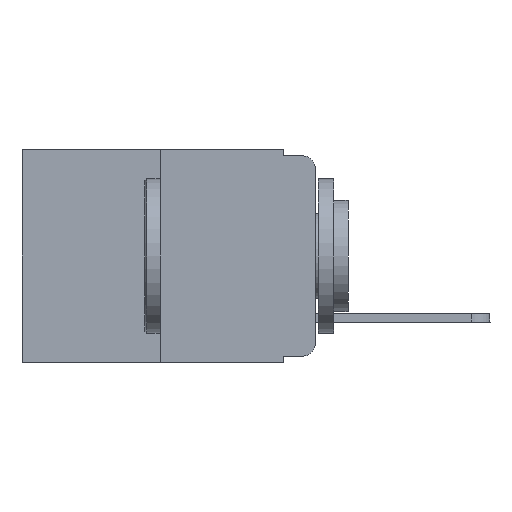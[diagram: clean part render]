
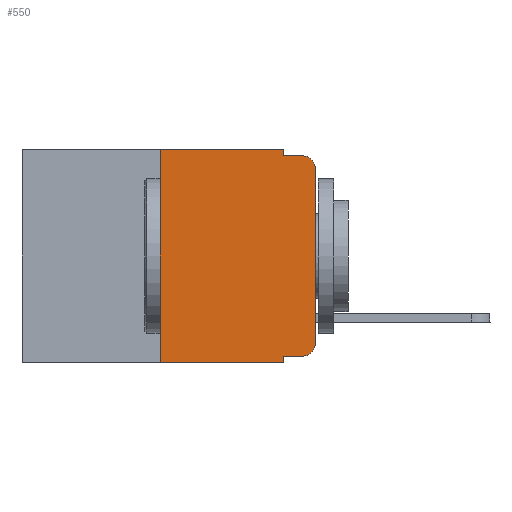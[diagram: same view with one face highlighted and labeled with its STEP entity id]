
A CAD part, left-side view. The second image highlights one B-rep face of the part: STEP entity #550.
In plain terms, the highlighted planar face has unit normal (-1, 0, 0).
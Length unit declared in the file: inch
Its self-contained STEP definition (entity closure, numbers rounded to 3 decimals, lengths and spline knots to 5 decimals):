
#314 = FACE_OUTER_BOUND ( 'NONE', #7585, .T. ) ;
#362 = DIRECTION ( 'NONE',  ( 0., 0., -1. ) ) ;
#365 = VERTEX_POINT ( 'NONE', #3191 ) ;
#460 = CIRCLE ( 'NONE', #5565, 0.02 ) ;
#550 = ADVANCED_FACE ( 'NONE', ( #314 ), #1403, .F. ) ;
#866 = DIRECTION ( 'NONE',  ( 0., 0., 1. ) ) ;
#910 = EDGE_CURVE ( 'NONE', #6566, #10781, #9144, .T. ) ;
#1000 = CARTESIAN_POINT ( 'NONE',  ( 0., 0.473, 0. ) ) ;
#1009 = EDGE_CURVE ( 'NONE', #2605, #8989, #460, .T. ) ;
#1221 = VERTEX_POINT ( 'NONE', #10163 ) ;
#1403 = PLANE ( 'NONE',  #7689 ) ;
#1728 = DIRECTION ( 'NONE',  ( 0., -1., 0. ) ) ;
#1851 = EDGE_CURVE ( 'NONE', #12961, #1221, #12371, .T. ) ;
#1961 = CARTESIAN_POINT ( 'NONE',  ( 0., 0.25, 0. ) ) ;
#2090 = DIRECTION ( 'NONE',  ( 0., -1., 0. ) ) ;
#2210 = VECTOR ( 'NONE', #2090, 39.37008 ) ;
#2278 = EDGE_CURVE ( 'NONE', #9634, #7809, #5179, .T. ) ;
#2605 = VERTEX_POINT ( 'NONE', #4623 ) ;
#2741 = CARTESIAN_POINT ( 'NONE',  ( 0., 0.473, -0.343 ) ) ;
#2773 = CARTESIAN_POINT ( 'NONE',  ( 0., 0.25, 0. ) ) ;
#2904 = CARTESIAN_POINT ( 'NONE',  ( 0., 0., -0.313 ) ) ;
#2907 = ORIENTED_EDGE ( 'NONE', *, *, #12034, .T. ) ;
#3114 = CARTESIAN_POINT ( 'NONE',  ( 0., 0.25, -0.343 ) ) ;
#3191 = CARTESIAN_POINT ( 'NONE',  ( 0., 0., -0.03 ) ) ;
#3356 = AXIS2_PLACEMENT_3D ( 'NONE', #10978, #5777, #4745 ) ;
#3427 = ORIENTED_EDGE ( 'NONE', *, *, #7143, .T. ) ;
#3485 = CARTESIAN_POINT ( 'NONE',  ( 0., 0.051, 0. ) ) ;
#3612 = DIRECTION ( 'NONE',  ( 0., 0., -1. ) ) ;
#3765 = ORIENTED_EDGE ( 'NONE', *, *, #4865, .F. ) ;
#3915 = LINE ( 'NONE', #3959, #11441 ) ;
#3959 = CARTESIAN_POINT ( 'NONE',  ( 0., 0.051, -0.333 ) ) ;
#4009 = CARTESIAN_POINT ( 'NONE',  ( 0., 0.051, 0. ) ) ;
#4623 = CARTESIAN_POINT ( 'NONE',  ( 0., 0.02, -0.333 ) ) ;
#4667 = DIRECTION ( 'NONE',  ( 1., 0., 0. ) ) ;
#4745 = DIRECTION ( 'NONE',  ( 0., 0., -1. ) ) ;
#4865 = EDGE_CURVE ( 'NONE', #7809, #6566, #5176, .T. ) ;
#5176 = LINE ( 'NONE', #1000, #2210 ) ;
#5179 = LINE ( 'NONE', #1961, #10401 ) ;
#5182 = ORIENTED_EDGE ( 'NONE', *, *, #1009, .T. ) ;
#5565 = AXIS2_PLACEMENT_3D ( 'NONE', #5571, #6618, #362 ) ;
#5571 = CARTESIAN_POINT ( 'NONE',  ( 0., 0.02, -0.313 ) ) ;
#5777 = DIRECTION ( 'NONE',  ( -1., 0., 0. ) ) ;
#5853 = VECTOR ( 'NONE', #6390, 39.37008 ) ;
#6011 = VECTOR ( 'NONE', #8711, 39.37008 ) ;
#6319 = VECTOR ( 'NONE', #11243, 39.37008 ) ;
#6356 = ORIENTED_EDGE ( 'NONE', *, *, #12206, .F. ) ;
#6390 = DIRECTION ( 'NONE',  ( 0., 0., 1. ) ) ;
#6396 = ORIENTED_EDGE ( 'NONE', *, *, #1851, .F. ) ;
#6566 = VERTEX_POINT ( 'NONE', #13171 ) ;
#6618 = DIRECTION ( 'NONE',  ( -1., 0., 0. ) ) ;
#6968 = ORIENTED_EDGE ( 'NONE', *, *, #10096, .T. ) ;
#7143 = EDGE_CURVE ( 'NONE', #365, #11783, #8053, .T. ) ;
#7462 = LINE ( 'NONE', #11970, #10920 ) ;
#7585 = EDGE_LOOP ( 'NONE', ( #2907, #3427, #6356, #13407, #3765, #7840, #6968, #6396, #12524, #5182 ) ) ;
#7689 = AXIS2_PLACEMENT_3D ( 'NONE', #11916, #4667, #3612 ) ;
#7809 = VERTEX_POINT ( 'NONE', #2773 ) ;
#7840 = ORIENTED_EDGE ( 'NONE', *, *, #2278, .F. ) ;
#8053 = CIRCLE ( 'NONE', #3356, 0.02 ) ;
#8711 = DIRECTION ( 'NONE',  ( 0., 0., -1. ) ) ;
#8807 = DIRECTION ( 'NONE',  ( 0., -1., 0. ) ) ;
#8965 = LINE ( 'NONE', #10591, #5853 ) ;
#8989 = VERTEX_POINT ( 'NONE', #2904 ) ;
#9144 = LINE ( 'NONE', #3485, #6011 ) ;
#9486 = EDGE_CURVE ( 'NONE', #12961, #2605, #3915, .T. ) ;
#9634 = VERTEX_POINT ( 'NONE', #3114 ) ;
#10067 = CARTESIAN_POINT ( 'NONE',  ( 0., 0.02, -0.01 ) ) ;
#10096 = EDGE_CURVE ( 'NONE', #9634, #1221, #10414, .T. ) ;
#10163 = CARTESIAN_POINT ( 'NONE',  ( 0., 0.051, -0.343 ) ) ;
#10401 = VECTOR ( 'NONE', #866, 39.37008 ) ;
#10414 = LINE ( 'NONE', #2741, #10738 ) ;
#10591 = CARTESIAN_POINT ( 'NONE',  ( 0., 0., 0. ) ) ;
#10738 = VECTOR ( 'NONE', #1728, 39.37008 ) ;
#10781 = VERTEX_POINT ( 'NONE', #11345 ) ;
#10920 = VECTOR ( 'NONE', #8807, 39.37008 ) ;
#10978 = CARTESIAN_POINT ( 'NONE',  ( 0., 0.02, -0.03 ) ) ;
#11082 = CARTESIAN_POINT ( 'NONE',  ( 0., 0.051, -0.333 ) ) ;
#11243 = DIRECTION ( 'NONE',  ( 0., 0., -1. ) ) ;
#11250 = DIRECTION ( 'NONE',  ( 0., -1., 0. ) ) ;
#11345 = CARTESIAN_POINT ( 'NONE',  ( 0., 0.051, -0.01 ) ) ;
#11441 = VECTOR ( 'NONE', #11250, 39.37008 ) ;
#11783 = VERTEX_POINT ( 'NONE', #10067 ) ;
#11916 = CARTESIAN_POINT ( 'NONE',  ( 0., 0.473, 0. ) ) ;
#11970 = CARTESIAN_POINT ( 'NONE',  ( 0., 0.051, -0.01 ) ) ;
#12034 = EDGE_CURVE ( 'NONE', #8989, #365, #8965, .T. ) ;
#12206 = EDGE_CURVE ( 'NONE', #10781, #11783, #7462, .T. ) ;
#12371 = LINE ( 'NONE', #4009, #6319 ) ;
#12524 = ORIENTED_EDGE ( 'NONE', *, *, #9486, .T. ) ;
#12961 = VERTEX_POINT ( 'NONE', #11082 ) ;
#13171 = CARTESIAN_POINT ( 'NONE',  ( 0., 0.051, 0. ) ) ;
#13407 = ORIENTED_EDGE ( 'NONE', *, *, #910, .F. ) ;
